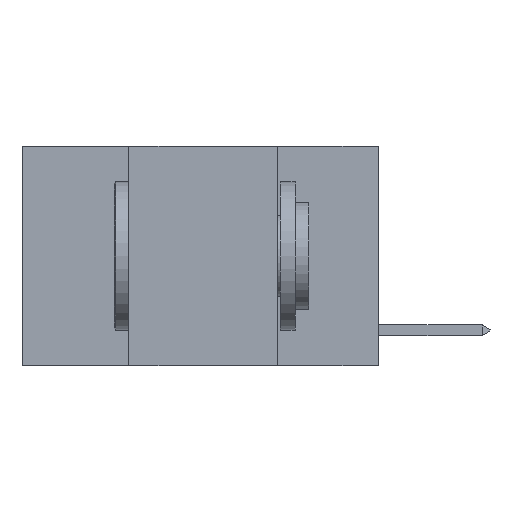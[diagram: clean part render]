
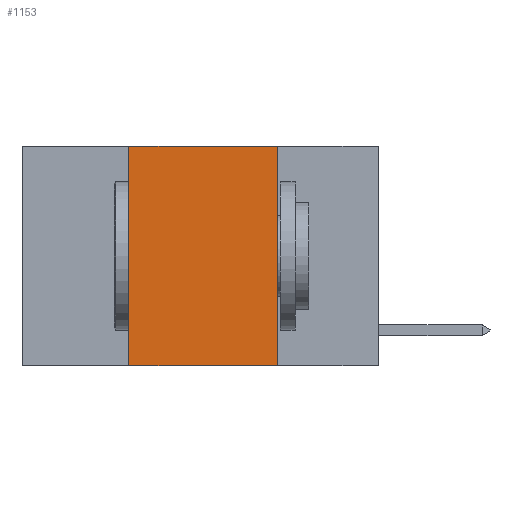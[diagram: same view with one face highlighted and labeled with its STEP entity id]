
A CAD part, left-side view. The second image highlights one B-rep face of the part: STEP entity #1153.
In plain terms, the highlighted planar face has unit normal (-1, 0, 0).
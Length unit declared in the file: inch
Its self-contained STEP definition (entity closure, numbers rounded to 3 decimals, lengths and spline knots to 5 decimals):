
#307 = CARTESIAN_POINT ( 'NONE',  ( 0., 0.42, 0. ) ) ;
#1153 = ADVANCED_FACE ( 'NONE', ( #2832 ), #6251, .F. ) ;
#1193 = VERTEX_POINT ( 'NONE', #1681 ) ;
#1655 = EDGE_CURVE ( 'NONE', #3192, #1193, #1868, .T. ) ;
#1681 = CARTESIAN_POINT ( 'NONE',  ( 0., 0.17, 0. ) ) ;
#1868 = LINE ( 'NONE', #7019, #9363 ) ;
#2448 = VERTEX_POINT ( 'NONE', #3401 ) ;
#2453 = VERTEX_POINT ( 'NONE', #4135 ) ;
#2649 = ORIENTED_EDGE ( 'NONE', *, *, #1655, .F. ) ;
#2832 = FACE_OUTER_BOUND ( 'NONE', #6556, .T. ) ;
#3192 = VERTEX_POINT ( 'NONE', #9268 ) ;
#3215 = CARTESIAN_POINT ( 'NONE',  ( 0., 0.17, 0. ) ) ;
#3401 = CARTESIAN_POINT ( 'NONE',  ( 0., 0.42, -0.37 ) ) ;
#3492 = LINE ( 'NONE', #3215, #7100 ) ;
#3559 = EDGE_CURVE ( 'NONE', #1193, #2453, #3492, .T. ) ;
#4135 = CARTESIAN_POINT ( 'NONE',  ( 0., 0.17, -0.37 ) ) ;
#4615 = LINE ( 'NONE', #9049, #6746 ) ;
#4748 = DIRECTION ( 'NONE',  ( 0., -1., 0. ) ) ;
#4921 = ORIENTED_EDGE ( 'NONE', *, *, #3559, .F. ) ;
#5092 = VECTOR ( 'NONE', #7678, 39.37008 ) ;
#5155 = ORIENTED_EDGE ( 'NONE', *, *, #5494, .F. ) ;
#5494 = EDGE_CURVE ( 'NONE', #2448, #3192, #7017, .T. ) ;
#6053 = DIRECTION ( 'NONE',  ( 1., 0., 0. ) ) ;
#6251 = PLANE ( 'NONE',  #7656 ) ;
#6430 = DIRECTION ( 'NONE',  ( 0., 0., -1. ) ) ;
#6556 = EDGE_LOOP ( 'NONE', ( #4921, #2649, #5155, #7445 ) ) ;
#6746 = VECTOR ( 'NONE', #4748, 39.37008 ) ;
#6757 = DIRECTION ( 'NONE',  ( 0., -1., 0. ) ) ;
#7017 = LINE ( 'NONE', #307, #5092 ) ;
#7019 = CARTESIAN_POINT ( 'NONE',  ( 0., 0.6, 0. ) ) ;
#7100 = VECTOR ( 'NONE', #8290, 39.37008 ) ;
#7445 = ORIENTED_EDGE ( 'NONE', *, *, #8411, .T. ) ;
#7573 = CARTESIAN_POINT ( 'NONE',  ( 0., 0.6, 0. ) ) ;
#7656 = AXIS2_PLACEMENT_3D ( 'NONE', #7573, #6053, #6430 ) ;
#7678 = DIRECTION ( 'NONE',  ( 0., 0., 1. ) ) ;
#8290 = DIRECTION ( 'NONE',  ( 0., 0., -1. ) ) ;
#8411 = EDGE_CURVE ( 'NONE', #2448, #2453, #4615, .T. ) ;
#9049 = CARTESIAN_POINT ( 'NONE',  ( 0., 0.6, -0.37 ) ) ;
#9268 = CARTESIAN_POINT ( 'NONE',  ( 0., 0.42, 0. ) ) ;
#9363 = VECTOR ( 'NONE', #6757, 39.37008 ) ;
